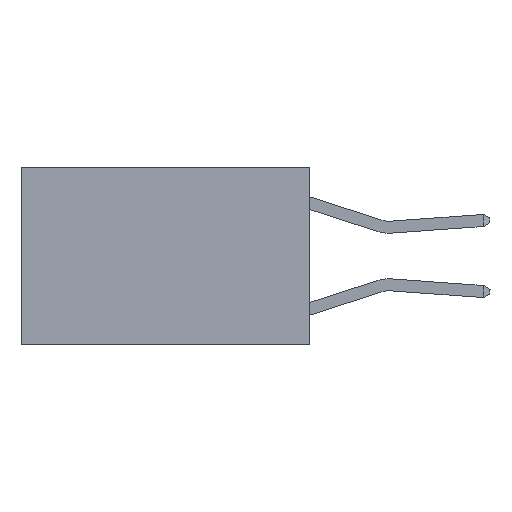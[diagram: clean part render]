
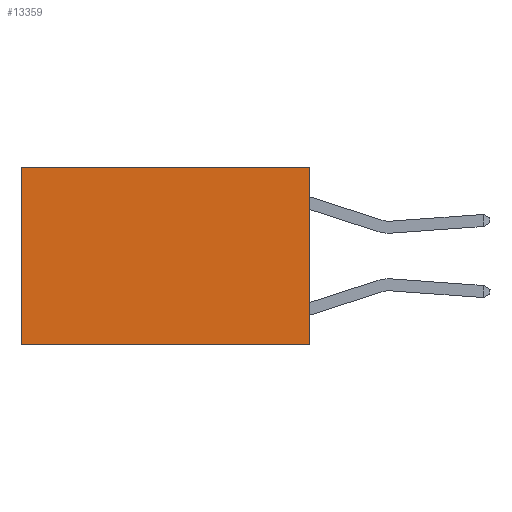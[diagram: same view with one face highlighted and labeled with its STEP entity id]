
A CAD part, left-side view. The second image highlights one B-rep face of the part: STEP entity #13359.
In plain terms, the highlighted planar face has unit normal (-1, 0, 0).
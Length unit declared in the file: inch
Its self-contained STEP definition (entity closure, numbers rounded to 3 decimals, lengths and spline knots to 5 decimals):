
#1756 = CARTESIAN_POINT ( 'NONE',  ( 0.2625, 0.6, 0. ) ) ;
#1835 = AXIS2_PLACEMENT_3D ( 'NONE', #11738, #13647, #2403 ) ;
#2403 = DIRECTION ( 'NONE',  ( 0., 0., -1. ) ) ;
#3218 = ORIENTED_EDGE ( 'NONE', *, *, #20875, .T. ) ;
#3661 = VECTOR ( 'NONE', #10130, 39.37008 ) ;
#5313 = FACE_OUTER_BOUND ( 'NONE', #23364, .T. ) ;
#6569 = DIRECTION ( 'NONE',  ( 0., 0., -1. ) ) ;
#7033 = VERTEX_POINT ( 'NONE', #1756 ) ;
#7309 = EDGE_CURVE ( 'NONE', #12721, #7033, #20754, .T. ) ;
#9258 = VERTEX_POINT ( 'NONE', #20706 ) ;
#9515 = CARTESIAN_POINT ( 'NONE',  ( 0.2625, 0., 0. ) ) ;
#9871 = PLANE ( 'NONE',  #1835 ) ;
#9899 = DIRECTION ( 'NONE',  ( 0., 1., 0. ) ) ;
#10065 = ORIENTED_EDGE ( 'NONE', *, *, #15834, .F. ) ;
#10130 = DIRECTION ( 'NONE',  ( 0., 1., 0. ) ) ;
#10865 = VECTOR ( 'NONE', #9899, 39.37008 ) ;
#11738 = CARTESIAN_POINT ( 'NONE',  ( 0.2625, 0., 0. ) ) ;
#11927 = CARTESIAN_POINT ( 'NONE',  ( 0.2625, 0., -0.37 ) ) ;
#12303 = LINE ( 'NONE', #19585, #22182 ) ;
#12721 = VERTEX_POINT ( 'NONE', #23730 ) ;
#13335 = LINE ( 'NONE', #9515, #23152 ) ;
#13359 = ADVANCED_FACE ( 'NONE', ( #5313 ), #9871, .F. ) ;
#13647 = DIRECTION ( 'NONE',  ( 1., 0., 0. ) ) ;
#13650 = LINE ( 'NONE', #11927, #3661 ) ;
#15515 = CARTESIAN_POINT ( 'NONE',  ( 0.2625, 0., 0. ) ) ;
#15834 = EDGE_CURVE ( 'NONE', #12721, #18008, #13335, .T. ) ;
#18008 = VERTEX_POINT ( 'NONE', #21606 ) ;
#19585 = CARTESIAN_POINT ( 'NONE',  ( 0.2625, 0.6, 0. ) ) ;
#20431 = ORIENTED_EDGE ( 'NONE', *, *, #23707, .F. ) ;
#20706 = CARTESIAN_POINT ( 'NONE',  ( 0.2625, 0.6, -0.37 ) ) ;
#20754 = LINE ( 'NONE', #15515, #10865 ) ;
#20875 = EDGE_CURVE ( 'NONE', #7033, #9258, #12303, .T. ) ;
#21606 = CARTESIAN_POINT ( 'NONE',  ( 0.2625, 0., -0.37 ) ) ;
#22182 = VECTOR ( 'NONE', #6569, 39.37008 ) ;
#22511 = DIRECTION ( 'NONE',  ( 0., 0., -1. ) ) ;
#22830 = ORIENTED_EDGE ( 'NONE', *, *, #7309, .T. ) ;
#23152 = VECTOR ( 'NONE', #22511, 39.37008 ) ;
#23364 = EDGE_LOOP ( 'NONE', ( #3218, #20431, #10065, #22830 ) ) ;
#23707 = EDGE_CURVE ( 'NONE', #18008, #9258, #13650, .T. ) ;
#23730 = CARTESIAN_POINT ( 'NONE',  ( 0.2625, 0., 0. ) ) ;
